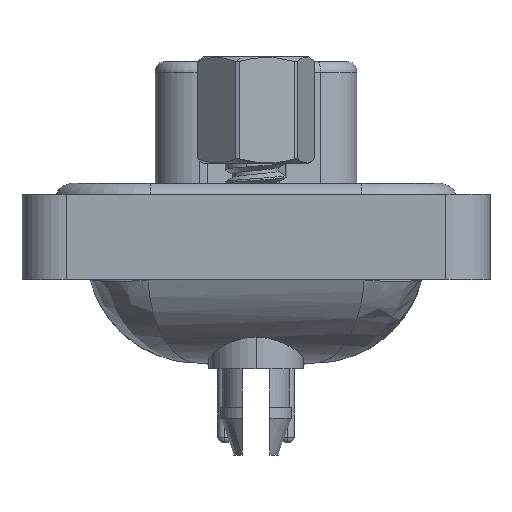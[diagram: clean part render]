
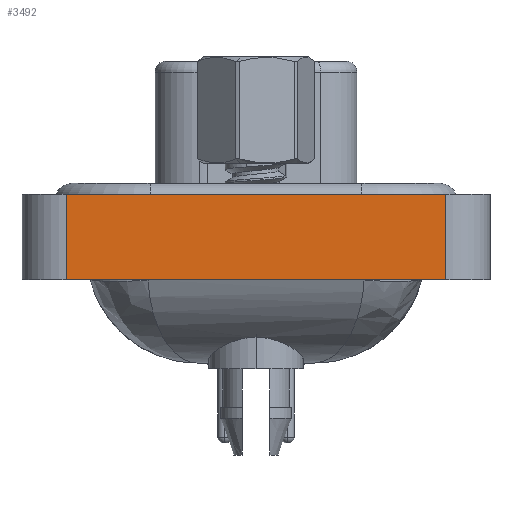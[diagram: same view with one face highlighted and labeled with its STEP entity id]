
A CAD part, left-side view. The second image highlights one B-rep face of the part: STEP entity #3492.
In plain terms, the highlighted planar face has unit normal (-1, 0, 0).
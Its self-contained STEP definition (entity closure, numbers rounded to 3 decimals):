
#264 = VECTOR ( 'NONE', #6960, 1000. ) ;
#454 = CARTESIAN_POINT ( 'NONE',  ( -7.35, 8.55, -3.35 ) ) ;
#867 = ORIENTED_EDGE ( 'NONE', *, *, #11966, .F. ) ;
#1146 = DIRECTION ( 'NONE',  ( 0., 0., 1. ) ) ;
#2279 = LINE ( 'NONE', #2397, #7846 ) ;
#2397 = CARTESIAN_POINT ( 'NONE',  ( -7.35, 8.55, -3.35 ) ) ;
#3492 = ADVANCED_FACE ( 'NONE', ( #15713 ), #11831, .T. ) ;
#4936 = CARTESIAN_POINT ( 'NONE',  ( -7.35, -8.55, 0.5 ) ) ;
#5118 = CARTESIAN_POINT ( 'NONE',  ( -7.35, -8.55, -3.35 ) ) ;
#5190 = VECTOR ( 'NONE', #22729, 1000. ) ;
#6172 = DIRECTION ( 'NONE',  ( 0., 0., 1. ) ) ;
#6250 = VERTEX_POINT ( 'NONE', #5118 ) ;
#6960 = DIRECTION ( 'NONE',  ( 0., 0., 1. ) ) ;
#7846 = VECTOR ( 'NONE', #6172, 1000. ) ;
#8724 = CARTESIAN_POINT ( 'NONE',  ( -7.35, -8.55, 0.5 ) ) ;
#8806 = CARTESIAN_POINT ( 'NONE',  ( -7.35, 8.55, 0.5 ) ) ;
#9835 = ORIENTED_EDGE ( 'NONE', *, *, #22857, .T. ) ;
#10280 = DIRECTION ( 'NONE',  ( 0., -1., 0. ) ) ;
#10946 = VERTEX_POINT ( 'NONE', #8806 ) ;
#11005 = VECTOR ( 'NONE', #10280, 1000. ) ;
#11132 = CARTESIAN_POINT ( 'NONE',  ( -7.35, -8.55, -3.35 ) ) ;
#11831 = PLANE ( 'NONE',  #20870 ) ;
#11944 = VERTEX_POINT ( 'NONE', #454 ) ;
#11966 = EDGE_CURVE ( 'NONE', #11944, #10946, #2279, .T. ) ;
#12860 = VERTEX_POINT ( 'NONE', #8724 ) ;
#14897 = EDGE_CURVE ( 'NONE', #11944, #6250, #17152, .T. ) ;
#15443 = ORIENTED_EDGE ( 'NONE', *, *, #17304, .F. ) ;
#15713 = FACE_OUTER_BOUND ( 'NONE', #21331, .T. ) ;
#17152 = LINE ( 'NONE', #11132, #5190 ) ;
#17304 = EDGE_CURVE ( 'NONE', #10946, #12860, #23747, .T. ) ;
#17776 = DIRECTION ( 'NONE',  ( -1., 0., 0. ) ) ;
#19444 = CARTESIAN_POINT ( 'NONE',  ( -7.35, -8.55, -3.35 ) ) ;
#19739 = ORIENTED_EDGE ( 'NONE', *, *, #14897, .T. ) ;
#20870 = AXIS2_PLACEMENT_3D ( 'NONE', #23112, #17776, #1146 ) ;
#21331 = EDGE_LOOP ( 'NONE', ( #9835, #15443, #867, #19739 ) ) ;
#22729 = DIRECTION ( 'NONE',  ( 0., -1., 0. ) ) ;
#22857 = EDGE_CURVE ( 'NONE', #6250, #12860, #23078, .T. ) ;
#23078 = LINE ( 'NONE', #19444, #264 ) ;
#23112 = CARTESIAN_POINT ( 'NONE',  ( -7.35, -8.55, -3.35 ) ) ;
#23747 = LINE ( 'NONE', #4936, #11005 ) ;
